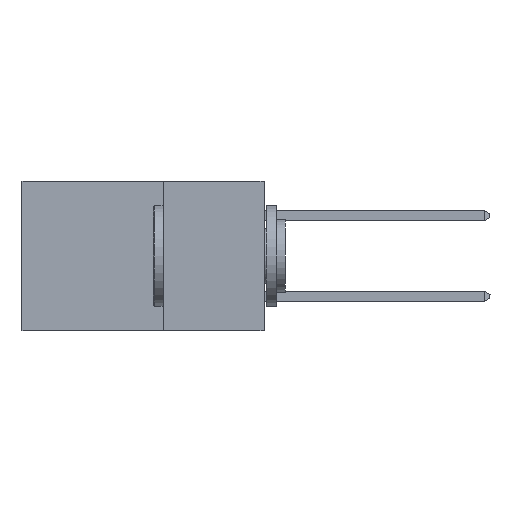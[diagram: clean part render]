
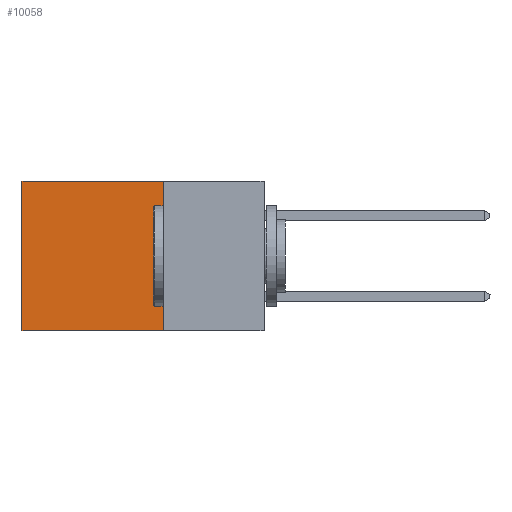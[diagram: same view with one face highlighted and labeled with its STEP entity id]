
A CAD part, left-side view. The second image highlights one B-rep face of the part: STEP entity #10058.
In plain terms, the highlighted planar face has unit normal (-1, 0, 0).
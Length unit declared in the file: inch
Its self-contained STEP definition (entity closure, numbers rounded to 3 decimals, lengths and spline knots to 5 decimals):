
#1022 = CARTESIAN_POINT ( 'NONE',  ( 0.298, 0.25, 0. ) ) ;
#1757 = AXIS2_PLACEMENT_3D ( 'NONE', #4244, #9960, #12721 ) ;
#1892 = LINE ( 'NONE', #11338, #10806 ) ;
#2798 = PLANE ( 'NONE',  #1757 ) ;
#2997 = ORIENTED_EDGE ( 'NONE', *, *, #4429, .T. ) ;
#3916 = CARTESIAN_POINT ( 'NONE',  ( 0.298, 0.6, -0.37 ) ) ;
#4244 = CARTESIAN_POINT ( 'NONE',  ( 0.298, 0.25, 0. ) ) ;
#4429 = EDGE_CURVE ( 'NONE', #12098, #17304, #18064, .T. ) ;
#4963 = EDGE_LOOP ( 'NONE', ( #5859, #6214, #9550, #2997 ) ) ;
#5859 = ORIENTED_EDGE ( 'NONE', *, *, #10491, .T. ) ;
#6214 = ORIENTED_EDGE ( 'NONE', *, *, #14033, .F. ) ;
#6532 = VECTOR ( 'NONE', #8125, 39.37008 ) ;
#7123 = DIRECTION ( 'NONE',  ( 0., 1., 0. ) ) ;
#7329 = DIRECTION ( 'NONE',  ( 0., 0., -1. ) ) ;
#7685 = CARTESIAN_POINT ( 'NONE',  ( 0.298, 0.25, -0.37 ) ) ;
#8125 = DIRECTION ( 'NONE',  ( 0., 1., 0. ) ) ;
#8544 = LINE ( 'NONE', #12946, #16066 ) ;
#8764 = VERTEX_POINT ( 'NONE', #3916 ) ;
#9550 = ORIENTED_EDGE ( 'NONE', *, *, #17594, .F. ) ;
#9684 = VERTEX_POINT ( 'NONE', #7685 ) ;
#9960 = DIRECTION ( 'NONE',  ( 1., 0., 0. ) ) ;
#10058 = ADVANCED_FACE ( 'NONE', ( #10996 ), #2798, .F. ) ;
#10491 = EDGE_CURVE ( 'NONE', #17304, #8764, #8544, .T. ) ;
#10806 = VECTOR ( 'NONE', #7329, 39.37008 ) ;
#10996 = FACE_OUTER_BOUND ( 'NONE', #4963, .T. ) ;
#11338 = CARTESIAN_POINT ( 'NONE',  ( 0.298, 0.25, 0. ) ) ;
#11633 = DIRECTION ( 'NONE',  ( 0., 0., -1. ) ) ;
#12098 = VERTEX_POINT ( 'NONE', #1022 ) ;
#12556 = CARTESIAN_POINT ( 'NONE',  ( 0.298, 0.6, 0. ) ) ;
#12721 = DIRECTION ( 'NONE',  ( 0., 0., -1. ) ) ;
#12946 = CARTESIAN_POINT ( 'NONE',  ( 0.298, 0.6, 0. ) ) ;
#13141 = VECTOR ( 'NONE', #7123, 39.37008 ) ;
#13787 = LINE ( 'NONE', #14164, #13141 ) ;
#14033 = EDGE_CURVE ( 'NONE', #9684, #8764, #13787, .T. ) ;
#14164 = CARTESIAN_POINT ( 'NONE',  ( 0.298, 0.25, -0.37 ) ) ;
#16066 = VECTOR ( 'NONE', #11633, 39.37008 ) ;
#17304 = VERTEX_POINT ( 'NONE', #12556 ) ;
#17594 = EDGE_CURVE ( 'NONE', #12098, #9684, #1892, .T. ) ;
#18064 = LINE ( 'NONE', #18142, #6532 ) ;
#18142 = CARTESIAN_POINT ( 'NONE',  ( 0.298, 0.25, 0. ) ) ;
